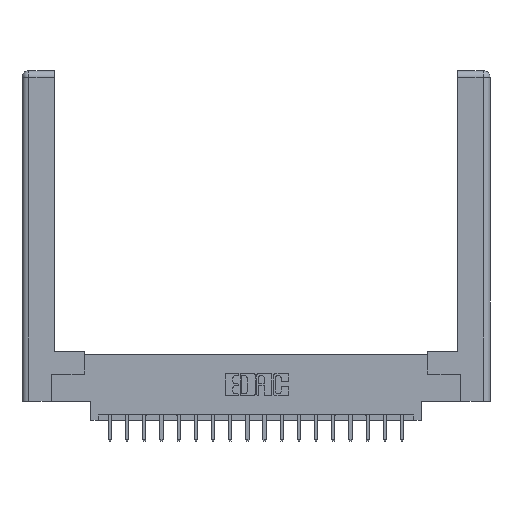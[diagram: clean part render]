
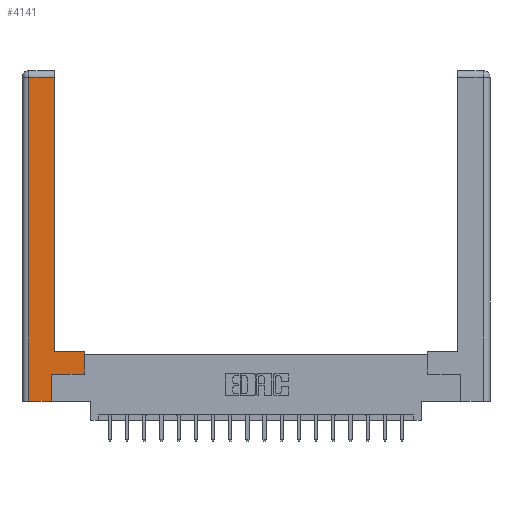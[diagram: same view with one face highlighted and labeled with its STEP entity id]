
A CAD part, top view. The second image highlights one B-rep face of the part: STEP entity #4141.
In plain terms, the highlighted planar face has unit normal (0, 0, 1).
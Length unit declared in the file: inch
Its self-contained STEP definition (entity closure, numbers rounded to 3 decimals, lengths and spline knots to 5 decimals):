
#55 = VECTOR ( 'NONE', #16749, 39.37008 ) ;
#176 = ORIENTED_EDGE ( 'NONE', *, *, #13927, .T. ) ;
#405 = VERTEX_POINT ( 'NONE', #19546 ) ;
#558 = EDGE_CURVE ( 'NONE', #8566, #405, #14583, .T. ) ;
#662 = DIRECTION ( 'NONE',  ( -1., 0., 0. ) ) ;
#1153 = CARTESIAN_POINT ( 'NONE',  ( 0.295, 0.45, 0. ) ) ;
#1486 = FACE_OUTER_BOUND ( 'NONE', #12384, .T. ) ;
#2014 = ORIENTED_EDGE ( 'NONE', *, *, #6762, .T. ) ;
#2655 = LINE ( 'NONE', #1153, #55 ) ;
#2703 = CARTESIAN_POINT ( 'NONE',  ( 0.265, 0., 0. ) ) ;
#2747 = CARTESIAN_POINT ( 'NONE',  ( 0.295, 0.45, 0. ) ) ;
#2866 = EDGE_CURVE ( 'NONE', #8643, #8566, #4159, .T. ) ;
#3031 = CARTESIAN_POINT ( 'NONE',  ( 0.265, 0., 0. ) ) ;
#3441 = ORIENTED_EDGE ( 'NONE', *, *, #558, .T. ) ;
#3826 = VERTEX_POINT ( 'NONE', #18031 ) ;
#4141 = ADVANCED_FACE ( 'NONE', ( #1486 ), #11451, .F. ) ;
#4159 = LINE ( 'NONE', #3031, #8783 ) ;
#4270 = CARTESIAN_POINT ( 'NONE',  ( 0.0615, 2.94, 0. ) ) ;
#4513 = DIRECTION ( 'NONE',  ( 1., 0., 0. ) ) ;
#4583 = VERTEX_POINT ( 'NONE', #11356 ) ;
#5362 = ORIENTED_EDGE ( 'NONE', *, *, #6997, .T. ) ;
#5588 = CARTESIAN_POINT ( 'NONE',  ( 0.0615, 0., 0. ) ) ;
#6083 = DIRECTION ( 'NONE',  ( -1., 0., 0. ) ) ;
#6108 = CARTESIAN_POINT ( 'NONE',  ( 0.295, 3., 0. ) ) ;
#6192 = LINE ( 'NONE', #11043, #10747 ) ;
#6311 = EDGE_CURVE ( 'NONE', #4583, #16286, #2655, .T. ) ;
#6451 = DIRECTION ( 'NONE',  ( 1., 0., 0. ) ) ;
#6653 = ORIENTED_EDGE ( 'NONE', *, *, #2866, .T. ) ;
#6762 = EDGE_CURVE ( 'NONE', #3826, #8080, #14217, .T. ) ;
#6997 = EDGE_CURVE ( 'NONE', #8080, #8643, #17105, .T. ) ;
#7017 = CARTESIAN_POINT ( 'NONE',  ( 0.265, 0.245, 0. ) ) ;
#7735 = DIRECTION ( 'NONE',  ( 0., 1., 0. ) ) ;
#8080 = VERTEX_POINT ( 'NONE', #4270 ) ;
#8566 = VERTEX_POINT ( 'NONE', #2703 ) ;
#8636 = AXIS2_PLACEMENT_3D ( 'NONE', #18916, #12882, #662 ) ;
#8643 = VERTEX_POINT ( 'NONE', #16648 ) ;
#8743 = EDGE_CURVE ( 'NONE', #405, #11926, #6192, .T. ) ;
#8783 = VECTOR ( 'NONE', #4513, 39.37008 ) ;
#9078 = ORIENTED_EDGE ( 'NONE', *, *, #15710, .T. ) ;
#9281 = CARTESIAN_POINT ( 'NONE',  ( 0.0615, 2.94, 0. ) ) ;
#9910 = VECTOR ( 'NONE', #6083, 39.37008 ) ;
#10017 = VECTOR ( 'NONE', #11365, 39.37008 ) ;
#10460 = ORIENTED_EDGE ( 'NONE', *, *, #8743, .T. ) ;
#10511 = VECTOR ( 'NONE', #14728, 39.37008 ) ;
#10747 = VECTOR ( 'NONE', #6451, 39.37008 ) ;
#11043 = CARTESIAN_POINT ( 'NONE',  ( 0.565, 0.245, 0. ) ) ;
#11356 = CARTESIAN_POINT ( 'NONE',  ( 0.565, 0.45, 0. ) ) ;
#11365 = DIRECTION ( 'NONE',  ( 0., 1., 0. ) ) ;
#11407 = LINE ( 'NONE', #15957, #10017 ) ;
#11451 = PLANE ( 'NONE',  #8636 ) ;
#11926 = VERTEX_POINT ( 'NONE', #19265 ) ;
#12384 = EDGE_LOOP ( 'NONE', ( #176, #2014, #5362, #6653, #3441, #10460, #9078, #17173 ) ) ;
#12882 = DIRECTION ( 'NONE',  ( 0., 0., -1. ) ) ;
#13927 = EDGE_CURVE ( 'NONE', #16286, #3826, #15845, .T. ) ;
#14217 = LINE ( 'NONE', #9281, #9910 ) ;
#14583 = LINE ( 'NONE', #7017, #10511 ) ;
#14728 = DIRECTION ( 'NONE',  ( 0., 1., 0. ) ) ;
#15710 = EDGE_CURVE ( 'NONE', #11926, #4583, #11407, .T. ) ;
#15845 = LINE ( 'NONE', #6108, #18288 ) ;
#15957 = CARTESIAN_POINT ( 'NONE',  ( 0.565, 0.45, 0. ) ) ;
#16286 = VERTEX_POINT ( 'NONE', #2747 ) ;
#16480 = DIRECTION ( 'NONE',  ( 0., -1., 0. ) ) ;
#16648 = CARTESIAN_POINT ( 'NONE',  ( 0.0615, 0., 0. ) ) ;
#16749 = DIRECTION ( 'NONE',  ( -1., 0., 0. ) ) ;
#17105 = LINE ( 'NONE', #5588, #17338 ) ;
#17173 = ORIENTED_EDGE ( 'NONE', *, *, #6311, .T. ) ;
#17338 = VECTOR ( 'NONE', #16480, 39.37008 ) ;
#18031 = CARTESIAN_POINT ( 'NONE',  ( 0.295, 2.94, 0. ) ) ;
#18288 = VECTOR ( 'NONE', #7735, 39.37008 ) ;
#18916 = CARTESIAN_POINT ( 'NONE',  ( 0., 0., 0. ) ) ;
#19265 = CARTESIAN_POINT ( 'NONE',  ( 0.565, 0.245, 0. ) ) ;
#19546 = CARTESIAN_POINT ( 'NONE',  ( 0.265, 0.245, 0. ) ) ;
